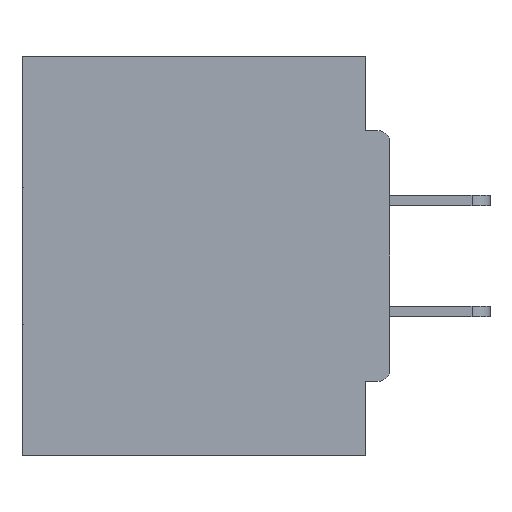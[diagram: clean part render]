
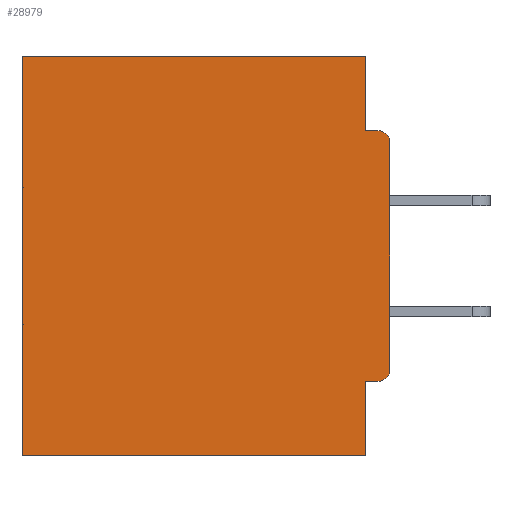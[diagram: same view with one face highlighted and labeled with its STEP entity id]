
A CAD part, left-side view. The second image highlights one B-rep face of the part: STEP entity #28979.
In plain terms, the highlighted planar face has unit normal (-1, 0, 0).
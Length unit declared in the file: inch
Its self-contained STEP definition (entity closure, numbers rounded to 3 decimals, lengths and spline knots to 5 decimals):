
#73 = VERTEX_POINT ( 'NONE', #38043 ) ;
#933 = ORIENTED_EDGE ( 'NONE', *, *, #2562, .F. ) ;
#2534 = ORIENTED_EDGE ( 'NONE', *, *, #16393, .F. ) ;
#2562 = EDGE_CURVE ( 'NONE', #21378, #29777, #37459, .T. ) ;
#2645 = DIRECTION ( 'NONE',  ( 0., 0., -1. ) ) ;
#3389 = PLANE ( 'NONE',  #33959 ) ;
#4619 = VERTEX_POINT ( 'NONE', #13085 ) ;
#5046 = CARTESIAN_POINT ( 'NONE',  ( 0.298, 0.031, -0.5 ) ) ;
#5293 = CARTESIAN_POINT ( 'NONE',  ( 0.298, 0.015, -0.1085 ) ) ;
#5512 = LINE ( 'NONE', #11476, #39997 ) ;
#6205 = CARTESIAN_POINT ( 'NONE',  ( 0.298, 0., -0.1085 ) ) ;
#6241 = CARTESIAN_POINT ( 'NONE',  ( 0.298, 0., 0. ) ) ;
#6561 = LINE ( 'NONE', #21624, #22107 ) ;
#7111 = EDGE_CURVE ( 'NONE', #36539, #4619, #31597, .T. ) ;
#7584 = EDGE_CURVE ( 'NONE', #18247, #16792, #20422, .T. ) ;
#8170 = EDGE_CURVE ( 'NONE', #40284, #36539, #27622, .T. ) ;
#9242 = CARTESIAN_POINT ( 'NONE',  ( 0.298, 0.015, -0.0935 ) ) ;
#11363 = CARTESIAN_POINT ( 'NONE',  ( 0.298, 0., -0.4065 ) ) ;
#11476 = CARTESIAN_POINT ( 'NONE',  ( 0.298, 0., -0.5 ) ) ;
#11724 = CARTESIAN_POINT ( 'NONE',  ( 0.298, 0.031, 0. ) ) ;
#12140 = VECTOR ( 'NONE', #38674, 39.37008 ) ;
#12216 = DIRECTION ( 'NONE',  ( 0., 0., -1. ) ) ;
#12250 = CARTESIAN_POINT ( 'NONE',  ( 0.298, 0.015, -0.4065 ) ) ;
#13009 = CARTESIAN_POINT ( 'NONE',  ( 0.298, 0.031, -0.4065 ) ) ;
#13062 = ORIENTED_EDGE ( 'NONE', *, *, #8170, .T. ) ;
#13085 = CARTESIAN_POINT ( 'NONE',  ( 0.298, 0.46, -0.5 ) ) ;
#13141 = CARTESIAN_POINT ( 'NONE',  ( 0.298, 0., 0. ) ) ;
#14659 = ORIENTED_EDGE ( 'NONE', *, *, #20513, .T. ) ;
#14690 = LINE ( 'NONE', #15246, #26893 ) ;
#15026 = DIRECTION ( 'NONE',  ( 0., 0., -1. ) ) ;
#15051 = CARTESIAN_POINT ( 'NONE',  ( 0.298, 0.031, -0.5 ) ) ;
#15246 = CARTESIAN_POINT ( 'NONE',  ( 0.298, 0.031, -0.5 ) ) ;
#15575 = DIRECTION ( 'NONE',  ( 0., 1., 0. ) ) ;
#15838 = DIRECTION ( 'NONE',  ( 1., 0., 0. ) ) ;
#16393 = EDGE_CURVE ( 'NONE', #29777, #4619, #5512, .T. ) ;
#16543 = CIRCLE ( 'NONE', #38433, 0.015 ) ;
#16792 = VERTEX_POINT ( 'NONE', #30513 ) ;
#17333 = CIRCLE ( 'NONE', #25355, 0.015 ) ;
#17342 = ORIENTED_EDGE ( 'NONE', *, *, #29498, .F. ) ;
#17454 = DIRECTION ( 'NONE',  ( 0., 1., 0. ) ) ;
#17462 = LINE ( 'NONE', #11363, #27197 ) ;
#18247 = VERTEX_POINT ( 'NONE', #6205 ) ;
#18504 = CARTESIAN_POINT ( 'NONE',  ( 0.298, 0.015, -0.3915 ) ) ;
#20422 = LINE ( 'NONE', #13141, #12140 ) ;
#20513 = EDGE_CURVE ( 'NONE', #24893, #16792, #17333, .T. ) ;
#21378 = VERTEX_POINT ( 'NONE', #13009 ) ;
#21624 = CARTESIAN_POINT ( 'NONE',  ( 0.298, 0., -0.0935 ) ) ;
#21889 = VECTOR ( 'NONE', #12216, 39.37008 ) ;
#22107 = VECTOR ( 'NONE', #39979, 39.37008 ) ;
#23432 = CARTESIAN_POINT ( 'NONE',  ( 0.298, 0.46, 0. ) ) ;
#23591 = ORIENTED_EDGE ( 'NONE', *, *, #36732, .F. ) ;
#24267 = EDGE_CURVE ( 'NONE', #73, #34130, #6561, .T. ) ;
#24850 = CARTESIAN_POINT ( 'NONE',  ( 0.298, 0., 0. ) ) ;
#24893 = VERTEX_POINT ( 'NONE', #12250 ) ;
#25355 = AXIS2_PLACEMENT_3D ( 'NONE', #18504, #40005, #31030 ) ;
#25451 = ORIENTED_EDGE ( 'NONE', *, *, #30593, .T. ) ;
#25997 = ORIENTED_EDGE ( 'NONE', *, *, #24267, .F. ) ;
#26545 = ORIENTED_EDGE ( 'NONE', *, *, #7584, .F. ) ;
#26893 = VECTOR ( 'NONE', #2645, 39.37008 ) ;
#27039 = DIRECTION ( 'NONE',  ( -1., 0., 0. ) ) ;
#27197 = VECTOR ( 'NONE', #17454, 39.37008 ) ;
#27622 = LINE ( 'NONE', #6241, #28603 ) ;
#28386 = DIRECTION ( 'NONE',  ( 0., 0., -1. ) ) ;
#28603 = VECTOR ( 'NONE', #15575, 39.37008 ) ;
#28979 = ADVANCED_FACE ( 'NONE', ( #31735 ), #3389, .F. ) ;
#29498 = EDGE_CURVE ( 'NONE', #40284, #73, #14690, .T. ) ;
#29693 = EDGE_LOOP ( 'NONE', ( #25451, #25997, #17342, #13062, #36768, #2534, #933, #23591, #14659, #26545 ) ) ;
#29777 = VERTEX_POINT ( 'NONE', #5046 ) ;
#30513 = CARTESIAN_POINT ( 'NONE',  ( 0.298, 0., -0.3915 ) ) ;
#30593 = EDGE_CURVE ( 'NONE', #18247, #34130, #16543, .T. ) ;
#31030 = DIRECTION ( 'NONE',  ( 0., 0., -1. ) ) ;
#31597 = LINE ( 'NONE', #32726, #37450 ) ;
#31735 = FACE_OUTER_BOUND ( 'NONE', #29693, .T. ) ;
#32193 = DIRECTION ( 'NONE',  ( 0., 0., -1. ) ) ;
#32726 = CARTESIAN_POINT ( 'NONE',  ( 0.298, 0.46, 0. ) ) ;
#33959 = AXIS2_PLACEMENT_3D ( 'NONE', #24850, #15838, #28386 ) ;
#34130 = VERTEX_POINT ( 'NONE', #9242 ) ;
#36539 = VERTEX_POINT ( 'NONE', #23432 ) ;
#36732 = EDGE_CURVE ( 'NONE', #24893, #21378, #17462, .T. ) ;
#36768 = ORIENTED_EDGE ( 'NONE', *, *, #7111, .T. ) ;
#37450 = VECTOR ( 'NONE', #32193, 39.37008 ) ;
#37459 = LINE ( 'NONE', #15051, #21889 ) ;
#38043 = CARTESIAN_POINT ( 'NONE',  ( 0.298, 0.031, -0.0935 ) ) ;
#38433 = AXIS2_PLACEMENT_3D ( 'NONE', #5293, #27039, #15026 ) ;
#38674 = DIRECTION ( 'NONE',  ( 0., 0., -1. ) ) ;
#39314 = DIRECTION ( 'NONE',  ( 0., 1., 0. ) ) ;
#39979 = DIRECTION ( 'NONE',  ( 0., -1., 0. ) ) ;
#39997 = VECTOR ( 'NONE', #39314, 39.37008 ) ;
#40005 = DIRECTION ( 'NONE',  ( -1., 0., 0. ) ) ;
#40284 = VERTEX_POINT ( 'NONE', #11724 ) ;
